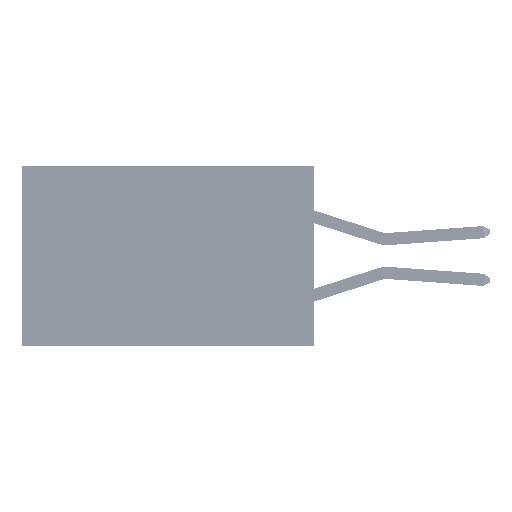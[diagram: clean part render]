
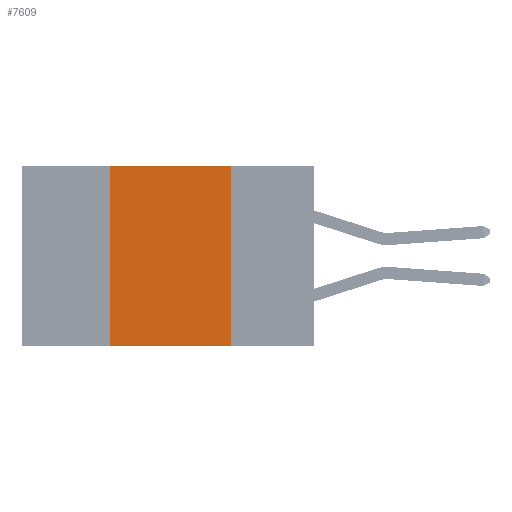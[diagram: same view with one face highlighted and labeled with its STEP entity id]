
A CAD part, left-side view. The second image highlights one B-rep face of the part: STEP entity #7609.
In plain terms, the highlighted planar face has unit normal (-1, 0, 0).
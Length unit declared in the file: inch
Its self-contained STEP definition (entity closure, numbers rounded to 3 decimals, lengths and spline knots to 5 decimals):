
#1446 = CARTESIAN_POINT ( 'NONE',  ( 0., 0.17, 0. ) ) ;
#2674 = DIRECTION ( 'NONE',  ( 0., 0., 1. ) ) ;
#2788 = VERTEX_POINT ( 'NONE', #5136 ) ;
#4026 = ORIENTED_EDGE ( 'NONE', *, *, #33646, .F. ) ;
#5136 = CARTESIAN_POINT ( 'NONE',  ( 0., 0.42, -0.37 ) ) ;
#5876 = EDGE_CURVE ( 'NONE', #2788, #28487, #16427, .T. ) ;
#6012 = EDGE_LOOP ( 'NONE', ( #4026, #12382, #29779, #41668 ) ) ;
#7609 = ADVANCED_FACE ( 'NONE', ( #23163 ), #46410, .F. ) ;
#12382 = ORIENTED_EDGE ( 'NONE', *, *, #42597, .F. ) ;
#12808 = DIRECTION ( 'NONE',  ( 0., -1., 0. ) ) ;
#12988 = CARTESIAN_POINT ( 'NONE',  ( 0., 0.6, 0. ) ) ;
#15491 = LINE ( 'NONE', #44822, #18962 ) ;
#16427 = LINE ( 'NONE', #45990, #25571 ) ;
#16428 = AXIS2_PLACEMENT_3D ( 'NONE', #12988, #23873, #34284 ) ;
#17188 = DIRECTION ( 'NONE',  ( 0., -1., 0. ) ) ;
#18962 = VECTOR ( 'NONE', #33411, 39.37008 ) ;
#20821 = CARTESIAN_POINT ( 'NONE',  ( 0., 0.42, 0. ) ) ;
#21120 = LINE ( 'NONE', #35878, #46209 ) ;
#21920 = VERTEX_POINT ( 'NONE', #20821 ) ;
#23163 = FACE_OUTER_BOUND ( 'NONE', #6012, .T. ) ;
#23873 = DIRECTION ( 'NONE',  ( 1., 0., 0. ) ) ;
#25571 = VECTOR ( 'NONE', #12808, 39.37008 ) ;
#27428 = CARTESIAN_POINT ( 'NONE',  ( 0., 0.17, -0.37 ) ) ;
#28487 = VERTEX_POINT ( 'NONE', #27428 ) ;
#29779 = ORIENTED_EDGE ( 'NONE', *, *, #36576, .F. ) ;
#33411 = DIRECTION ( 'NONE',  ( 0., 0., -1. ) ) ;
#33646 = EDGE_CURVE ( 'NONE', #41026, #28487, #15491, .T. ) ;
#34284 = DIRECTION ( 'NONE',  ( 0., 0., -1. ) ) ;
#35569 = CARTESIAN_POINT ( 'NONE',  ( 0., 0.6, 0. ) ) ;
#35878 = CARTESIAN_POINT ( 'NONE',  ( 0., 0.42, 0. ) ) ;
#36576 = EDGE_CURVE ( 'NONE', #2788, #21920, #21120, .T. ) ;
#39948 = LINE ( 'NONE', #35569, #44925 ) ;
#41026 = VERTEX_POINT ( 'NONE', #1446 ) ;
#41668 = ORIENTED_EDGE ( 'NONE', *, *, #5876, .T. ) ;
#42597 = EDGE_CURVE ( 'NONE', #21920, #41026, #39948, .T. ) ;
#44822 = CARTESIAN_POINT ( 'NONE',  ( 0., 0.17, 0. ) ) ;
#44925 = VECTOR ( 'NONE', #17188, 39.37008 ) ;
#45990 = CARTESIAN_POINT ( 'NONE',  ( 0., 0.6, -0.37 ) ) ;
#46209 = VECTOR ( 'NONE', #2674, 39.37008 ) ;
#46410 = PLANE ( 'NONE',  #16428 ) ;
